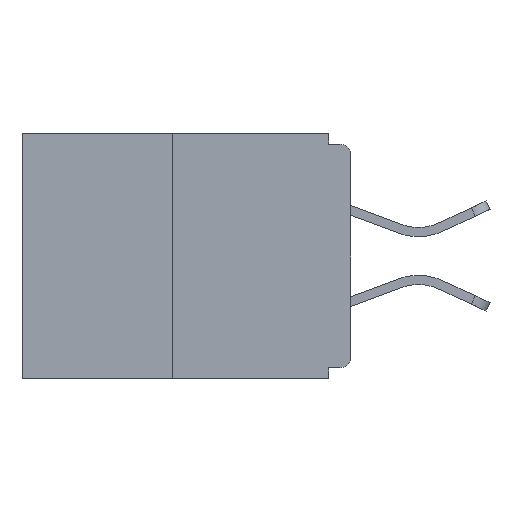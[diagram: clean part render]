
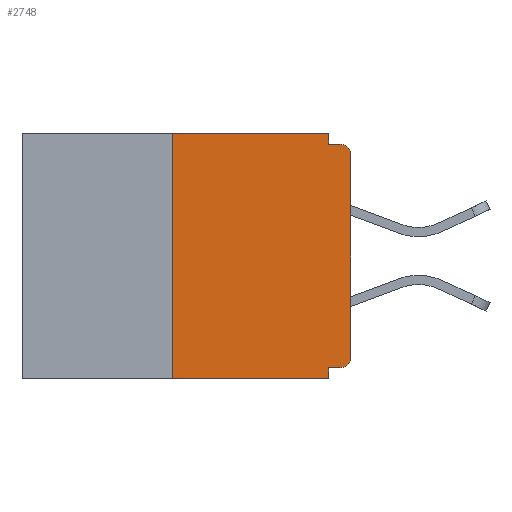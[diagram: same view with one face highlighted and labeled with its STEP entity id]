
A CAD part, left-side view. The second image highlights one B-rep face of the part: STEP entity #2748.
In plain terms, the highlighted planar face has unit normal (-1, 0, 0).
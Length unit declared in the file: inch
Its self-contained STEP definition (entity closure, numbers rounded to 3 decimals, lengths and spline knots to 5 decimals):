
#428 = DIRECTION ( 'NONE',  ( 0., 0., -1. ) ) ;
#871 = CARTESIAN_POINT ( 'NONE',  ( 0., 0.46, -0.343 ) ) ;
#949 = CARTESIAN_POINT ( 'NONE',  ( 0., 0.031, -0.343 ) ) ;
#1147 = VERTEX_POINT ( 'NONE', #13602 ) ;
#1242 = VECTOR ( 'NONE', #1753, 39.37008 ) ;
#1282 = CARTESIAN_POINT ( 'NONE',  ( 0., 0.46, 0. ) ) ;
#1375 = DIRECTION ( 'NONE',  ( -1., 0., 0. ) ) ;
#1644 = CARTESIAN_POINT ( 'NONE',  ( 0., 0.25, 0. ) ) ;
#1658 = PLANE ( 'NONE',  #9369 ) ;
#1753 = DIRECTION ( 'NONE',  ( 0., 0., -1. ) ) ;
#1792 = CARTESIAN_POINT ( 'NONE',  ( 0., 0., -0.328 ) ) ;
#1994 = CARTESIAN_POINT ( 'NONE',  ( 0., 0.25, 0. ) ) ;
#2278 = ORIENTED_EDGE ( 'NONE', *, *, #11852, .F. ) ;
#2314 = EDGE_CURVE ( 'NONE', #14251, #13169, #4923, .T. ) ;
#2421 = VERTEX_POINT ( 'NONE', #6915 ) ;
#2438 = EDGE_CURVE ( 'NONE', #13169, #1147, #5576, .T. ) ;
#2497 = DIRECTION ( 'NONE',  ( -1., 0., 0. ) ) ;
#2748 = ADVANCED_FACE ( 'NONE', ( #8120 ), #1658, .F. ) ;
#2947 = VERTEX_POINT ( 'NONE', #15789 ) ;
#3562 = CARTESIAN_POINT ( 'NONE',  ( 0., 0., -0.015 ) ) ;
#3982 = ORIENTED_EDGE ( 'NONE', *, *, #12270, .F. ) ;
#4085 = EDGE_CURVE ( 'NONE', #13551, #12434, #14902, .T. ) ;
#4643 = DIRECTION ( 'NONE',  ( 0., 0., 1. ) ) ;
#4732 = LINE ( 'NONE', #1994, #10105 ) ;
#4882 = VECTOR ( 'NONE', #8561, 39.37008 ) ;
#4923 = LINE ( 'NONE', #1282, #9425 ) ;
#5196 = VECTOR ( 'NONE', #12527, 39.37008 ) ;
#5389 = CARTESIAN_POINT ( 'NONE',  ( 0., 0.46, 0. ) ) ;
#5499 = AXIS2_PLACEMENT_3D ( 'NONE', #12703, #1375, #8743 ) ;
#5576 = LINE ( 'NONE', #15645, #1242 ) ;
#5997 = DIRECTION ( 'NONE',  ( 0., 0., -1. ) ) ;
#6411 = CIRCLE ( 'NONE', #13517, 0.015 ) ;
#6478 = CARTESIAN_POINT ( 'NONE',  ( 0., 0.015, -0.313 ) ) ;
#6915 = CARTESIAN_POINT ( 'NONE',  ( 0., 0.015, -0.015 ) ) ;
#6977 = ORIENTED_EDGE ( 'NONE', *, *, #12334, .F. ) ;
#7019 = ORIENTED_EDGE ( 'NONE', *, *, #8497, .T. ) ;
#7314 = CARTESIAN_POINT ( 'NONE',  ( 0., 0.25, -0.343 ) ) ;
#7560 = DIRECTION ( 'NONE',  ( 0., 0., -1. ) ) ;
#7620 = CIRCLE ( 'NONE', #5499, 0.015 ) ;
#7807 = ORIENTED_EDGE ( 'NONE', *, *, #8873, .T. ) ;
#8031 = VERTEX_POINT ( 'NONE', #10394 ) ;
#8120 = FACE_OUTER_BOUND ( 'NONE', #15775, .T. ) ;
#8465 = LINE ( 'NONE', #3562, #9315 ) ;
#8497 = EDGE_CURVE ( 'NONE', #14142, #2421, #7620, .T. ) ;
#8561 = DIRECTION ( 'NONE',  ( 0., -1., 0. ) ) ;
#8626 = DIRECTION ( 'NONE',  ( 0., -1., 0. ) ) ;
#8668 = VECTOR ( 'NONE', #11885, 39.37008 ) ;
#8743 = DIRECTION ( 'NONE',  ( 0., 0., -1. ) ) ;
#8873 = EDGE_CURVE ( 'NONE', #8031, #14142, #15071, .T. ) ;
#9117 = DIRECTION ( 'NONE',  ( 1., 0., 0. ) ) ;
#9259 = ORIENTED_EDGE ( 'NONE', *, *, #13661, .T. ) ;
#9315 = VECTOR ( 'NONE', #8626, 39.37008 ) ;
#9369 = AXIS2_PLACEMENT_3D ( 'NONE', #5389, #9117, #428 ) ;
#9425 = VECTOR ( 'NONE', #10201, 39.37008 ) ;
#10105 = VECTOR ( 'NONE', #4643, 39.37008 ) ;
#10201 = DIRECTION ( 'NONE',  ( 0., -1., 0. ) ) ;
#10394 = CARTESIAN_POINT ( 'NONE',  ( 0., 0., -0.313 ) ) ;
#10929 = EDGE_CURVE ( 'NONE', #2947, #14108, #13112, .T. ) ;
#11011 = ORIENTED_EDGE ( 'NONE', *, *, #10929, .F. ) ;
#11359 = CARTESIAN_POINT ( 'NONE',  ( 0., 0., 0. ) ) ;
#11773 = ORIENTED_EDGE ( 'NONE', *, *, #2314, .F. ) ;
#11852 = EDGE_CURVE ( 'NONE', #14108, #12434, #14906, .T. ) ;
#11885 = DIRECTION ( 'NONE',  ( 0., 1., 0. ) ) ;
#12270 = EDGE_CURVE ( 'NONE', #13551, #14251, #4732, .T. ) ;
#12334 = EDGE_CURVE ( 'NONE', #1147, #2421, #8465, .T. ) ;
#12434 = VERTEX_POINT ( 'NONE', #15059 ) ;
#12527 = DIRECTION ( 'NONE',  ( 0., 0., 1. ) ) ;
#12581 = CARTESIAN_POINT ( 'NONE',  ( 0., 0.031, -0.328 ) ) ;
#12703 = CARTESIAN_POINT ( 'NONE',  ( 0., 0.015, -0.03 ) ) ;
#13112 = LINE ( 'NONE', #1792, #8668 ) ;
#13169 = VERTEX_POINT ( 'NONE', #13580 ) ;
#13517 = AXIS2_PLACEMENT_3D ( 'NONE', #6478, #2497, #7560 ) ;
#13551 = VERTEX_POINT ( 'NONE', #7314 ) ;
#13580 = CARTESIAN_POINT ( 'NONE',  ( 0., 0.031, 0. ) ) ;
#13602 = CARTESIAN_POINT ( 'NONE',  ( 0., 0.031, -0.015 ) ) ;
#13661 = EDGE_CURVE ( 'NONE', #2947, #8031, #6411, .T. ) ;
#13874 = CARTESIAN_POINT ( 'NONE',  ( 0., 0., -0.03 ) ) ;
#14108 = VERTEX_POINT ( 'NONE', #12581 ) ;
#14117 = ORIENTED_EDGE ( 'NONE', *, *, #2438, .F. ) ;
#14142 = VERTEX_POINT ( 'NONE', #13874 ) ;
#14251 = VERTEX_POINT ( 'NONE', #1644 ) ;
#14301 = VECTOR ( 'NONE', #5997, 39.37008 ) ;
#14326 = ORIENTED_EDGE ( 'NONE', *, *, #4085, .T. ) ;
#14902 = LINE ( 'NONE', #871, #4882 ) ;
#14906 = LINE ( 'NONE', #949, #14301 ) ;
#15059 = CARTESIAN_POINT ( 'NONE',  ( 0., 0.031, -0.343 ) ) ;
#15071 = LINE ( 'NONE', #11359, #5196 ) ;
#15645 = CARTESIAN_POINT ( 'NONE',  ( 0., 0.031, 0. ) ) ;
#15775 = EDGE_LOOP ( 'NONE', ( #11773, #3982, #14326, #2278, #11011, #9259, #7807, #7019, #6977, #14117 ) ) ;
#15789 = CARTESIAN_POINT ( 'NONE',  ( 0., 0.015, -0.328 ) ) ;
